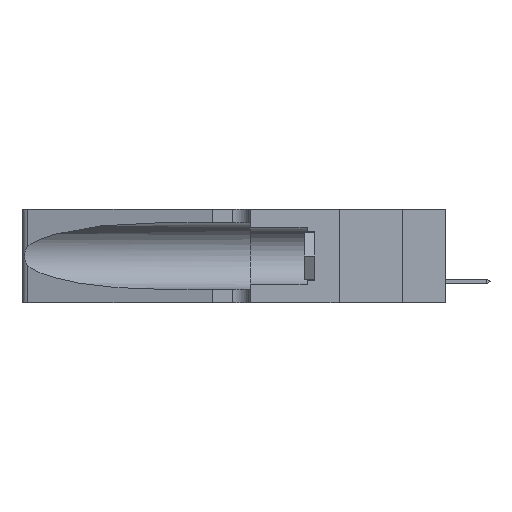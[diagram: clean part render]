
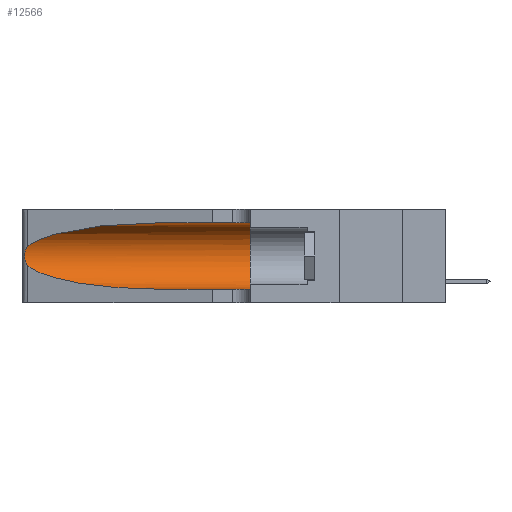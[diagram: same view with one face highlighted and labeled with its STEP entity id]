
A CAD part, left-side view. The second image highlights one B-rep face of the part: STEP entity #12566.
In plain terms, the highlighted cylindrical face has radius 3.308 mm (diameter 6.617 mm), a partial arc.
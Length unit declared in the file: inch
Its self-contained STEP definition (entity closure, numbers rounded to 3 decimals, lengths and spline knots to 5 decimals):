
#621 = VERTEX_POINT ( 'NONE', #17943 ) ;
#1163 = CARTESIAN_POINT ( 'NONE',  ( 0.26018, 1.23835, 0.19895 ) ) ;
#1348 = EDGE_CURVE ( 'NONE', #8926, #621, #14985, .T. ) ;
#1751 = CARTESIAN_POINT ( 'NONE',  ( 0.2373, 1.15595, 0.28018 ) ) ;
#2481 = EDGE_LOOP ( 'NONE', ( #16511, #22564, #18651, #2701, #20557, #12997 ) ) ;
#2701 = ORIENTED_EDGE ( 'NONE', *, *, #22927, .T. ) ;
#2952 = CARTESIAN_POINT ( 'NONE',  ( 0.25639, 1.23186, 0.15144 ) ) ;
#3232 = CARTESIAN_POINT ( 'NONE',  ( 0.26075, 1.23896, 0.178 ) ) ;
#3905 = CARTESIAN_POINT ( 'NONE',  ( 0.1305, 0.72297, 0.31525 ) ) ;
#4192 =( BOUNDED_CURVE ( )  B_SPLINE_CURVE ( 3, ( #21052, #14019, #21136, #16468 ),
 .UNSPECIFIED., .F., .F. ) 
 B_SPLINE_CURVE_WITH_KNOTS ( ( 4, 4 ),
 ( 3.44316, 4.71239 ),
 .UNSPECIFIED. ) 
 CURVE ( )  GEOMETRIC_REPRESENTATION_ITEM ( )  RATIONAL_B_SPLINE_CURVE ( ( 1., 0.87, 0.87, 1. ) ) 
 REPRESENTATION_ITEM ( '' )  );
#5480 = CARTESIAN_POINT ( 'NONE',  ( 0.25555, 1.22993, 0.14849 ) ) ;
#5796 =( BOUNDED_CURVE ( )  B_SPLINE_CURVE ( 3, ( #3905, #15182, #1751, #24282 ),
 .UNSPECIFIED., .F., .F. ) 
 B_SPLINE_CURVE_WITH_KNOTS ( ( 4, 4 ),
 ( 1.5708, 2.84003 ),
 .UNSPECIFIED. ) 
 CURVE ( )  GEOMETRIC_REPRESENTATION_ITEM ( )  RATIONAL_B_SPLINE_CURVE ( ( 1., 0.87, 0.87, 1. ) ) 
 REPRESENTATION_ITEM ( '' )  );
#6325 = DIRECTION ( 'NONE',  ( 0., 0., -1. ) ) ;
#7327 = VERTEX_POINT ( 'NONE', #9412 ) ;
#7509 = CARTESIAN_POINT ( 'NONE',  ( 0.25487, 1.22718, 0.22369 ) ) ;
#7602 = CARTESIAN_POINT ( 'NONE',  ( 0.25555, 1.22994, 0.2215 ) ) ;
#8365 = EDGE_CURVE ( 'NONE', #26275, #27285, #10396, .T. ) ;
#8366 = CARTESIAN_POINT ( 'NONE',  ( 0.1305, 1.61858, 0.185 ) ) ;
#8671 = VECTOR ( 'NONE', #9679, 39.37008 ) ;
#8926 = VERTEX_POINT ( 'NONE', #21718 ) ;
#9412 = CARTESIAN_POINT ( 'NONE',  ( 0.1305, 0.72297, 0.05475 ) ) ;
#9679 = DIRECTION ( 'NONE',  ( 0., -1., 0. ) ) ;
#9770 = CARTESIAN_POINT ( 'NONE',  ( 0.25856, 1.23593, 0.16098 ) ) ;
#10085 = CARTESIAN_POINT ( 'NONE',  ( 0.1305, 0.35, 0.31525 ) ) ;
#10218 = FACE_OUTER_BOUND ( 'NONE', #2481, .T. ) ;
#10396 = LINE ( 'NONE', #11053, #24776 ) ;
#11053 = CARTESIAN_POINT ( 'NONE',  ( 0.1305, 1.61858, 0.31525 ) ) ;
#11439 = CARTESIAN_POINT ( 'NONE',  ( 0.1305, 0.35, 0.185 ) ) ;
#12427 = CARTESIAN_POINT ( 'NONE',  ( 0.1305, 0.72297, 0.31525 ) ) ;
#12566 = ADVANCED_FACE ( 'NONE', ( #10218 ), #24606, .F. ) ;
#12997 = ORIENTED_EDGE ( 'NONE', *, *, #8365, .F. ) ;
#13408 = DIRECTION ( 'NONE',  ( 0., -1., 0. ) ) ;
#13697 = DIRECTION ( 'NONE',  ( 0., 1., 0. ) ) ;
#14019 = CARTESIAN_POINT ( 'NONE',  ( 0.2373, 1.15595, 0.08982 ) ) ;
#14493 = CARTESIAN_POINT ( 'NONE',  ( 0.26017, 1.23833, 0.17102 ) ) ;
#14666 = LINE ( 'NONE', #25784, #8671 ) ;
#14985 = B_SPLINE_CURVE_WITH_KNOTS ( 'NONE', 3,
 ( #7509, #7602, #18732, #25590, #16673, #1163, #23336, #3232, #14493, #9770, #16482, #2952, #5480, #21151 ),
 .UNSPECIFIED., .F., .F.,
 ( 4, 2, 2, 2, 2, 2, 4 ),
 ( 0., 0.00027, 0.00053, 0.00107, 0.0016, 0.00187, 0.00214 ),
 .UNSPECIFIED. ) ;
#15008 = AXIS2_PLACEMENT_3D ( 'NONE', #8366, #21849, #6325 ) ;
#15182 = CARTESIAN_POINT ( 'NONE',  ( 0.18966, 0.96281, 0.31525 ) ) ;
#15667 = DIRECTION ( 'NONE',  ( 0., 0., 1. ) ) ;
#16468 = CARTESIAN_POINT ( 'NONE',  ( 0.1305, 0.72297, 0.05475 ) ) ;
#16482 = CARTESIAN_POINT ( 'NONE',  ( 0.25789, 1.23486, 0.15765 ) ) ;
#16511 = ORIENTED_EDGE ( 'NONE', *, *, #26400, .T. ) ;
#16673 = CARTESIAN_POINT ( 'NONE',  ( 0.25854, 1.2359, 0.20912 ) ) ;
#17943 = CARTESIAN_POINT ( 'NONE',  ( 0.25487, 1.22718, 0.14631 ) ) ;
#18651 = ORIENTED_EDGE ( 'NONE', *, *, #28750, .T. ) ;
#18732 = CARTESIAN_POINT ( 'NONE',  ( 0.25639, 1.23184, 0.21858 ) ) ;
#20557 = ORIENTED_EDGE ( 'NONE', *, *, #26489, .F. ) ;
#21052 = CARTESIAN_POINT ( 'NONE',  ( 0.25487, 1.22718, 0.14631 ) ) ;
#21136 = CARTESIAN_POINT ( 'NONE',  ( 0.18966, 0.96281, 0.05475 ) ) ;
#21151 = CARTESIAN_POINT ( 'NONE',  ( 0.25487, 1.22718, 0.14631 ) ) ;
#21718 = CARTESIAN_POINT ( 'NONE',  ( 0.25487, 1.22718, 0.22369 ) ) ;
#21849 = DIRECTION ( 'NONE',  ( 0., -1., 0. ) ) ;
#22564 = ORIENTED_EDGE ( 'NONE', *, *, #1348, .T. ) ;
#22576 = AXIS2_PLACEMENT_3D ( 'NONE', #11439, #13697, #15667 ) ;
#22792 = CARTESIAN_POINT ( 'NONE',  ( 0.1305, 0.35, 0.05475 ) ) ;
#22927 = EDGE_CURVE ( 'NONE', #7327, #27207, #14666, .T. ) ;
#23336 = CARTESIAN_POINT ( 'NONE',  ( 0.26075, 1.23896, 0.19203 ) ) ;
#24282 = CARTESIAN_POINT ( 'NONE',  ( 0.25487, 1.22718, 0.22369 ) ) ;
#24387 = CIRCLE ( 'NONE', #22576, 0.13025 ) ;
#24606 = CYLINDRICAL_SURFACE ( 'NONE', #15008, 0.13025 ) ;
#24776 = VECTOR ( 'NONE', #13408, 39.37008 ) ;
#25590 = CARTESIAN_POINT ( 'NONE',  ( 0.25787, 1.23484, 0.2124 ) ) ;
#25784 = CARTESIAN_POINT ( 'NONE',  ( 0.1305, 1.61858, 0.05475 ) ) ;
#26275 = VERTEX_POINT ( 'NONE', #12427 ) ;
#26400 = EDGE_CURVE ( 'NONE', #26275, #8926, #5796, .T. ) ;
#26489 = EDGE_CURVE ( 'NONE', #27285, #27207, #24387, .T. ) ;
#27207 = VERTEX_POINT ( 'NONE', #22792 ) ;
#27285 = VERTEX_POINT ( 'NONE', #10085 ) ;
#28750 = EDGE_CURVE ( 'NONE', #621, #7327, #4192, .T. ) ;
